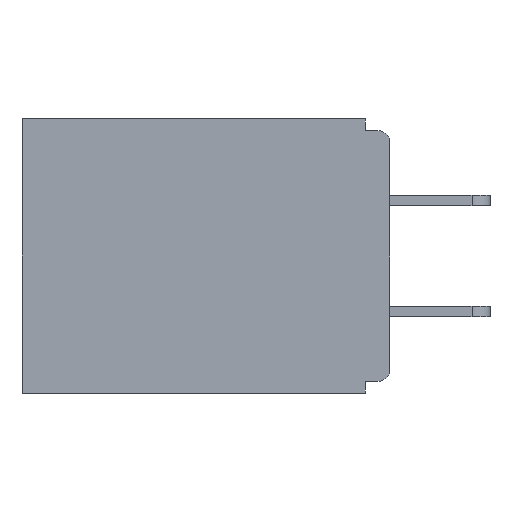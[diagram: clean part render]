
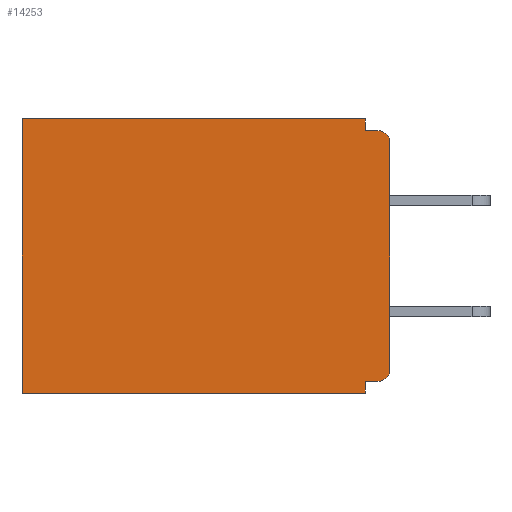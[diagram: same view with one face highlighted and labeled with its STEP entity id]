
A CAD part, left-side view. The second image highlights one B-rep face of the part: STEP entity #14253.
In plain terms, the highlighted planar face has unit normal (-1, 0, 0).
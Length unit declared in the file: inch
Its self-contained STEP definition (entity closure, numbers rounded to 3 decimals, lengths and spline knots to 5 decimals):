
#71 = VECTOR ( 'NONE', #6098, 39.37008 ) ;
#136 = LINE ( 'NONE', #7848, #893 ) ;
#165 = VECTOR ( 'NONE', #1914, 39.37008 ) ;
#212 = CARTESIAN_POINT ( 'NONE',  ( 0.298, 0.015, -0.313 ) ) ;
#882 = ORIENTED_EDGE ( 'NONE', *, *, #3048, .T. ) ;
#893 = VECTOR ( 'NONE', #1879, 39.37008 ) ;
#939 = EDGE_CURVE ( 'NONE', #12986, #13128, #13913, .T. ) ;
#944 = VERTEX_POINT ( 'NONE', #994 ) ;
#994 = CARTESIAN_POINT ( 'NONE',  ( 0.298, 0.031, 0. ) ) ;
#1046 = EDGE_CURVE ( 'NONE', #944, #14890, #9510, .T. ) ;
#1520 = CARTESIAN_POINT ( 'NONE',  ( 0.298, 0.46, 0. ) ) ;
#1879 = DIRECTION ( 'NONE',  ( 0., 0., -1. ) ) ;
#1914 = DIRECTION ( 'NONE',  ( 0., 1., 0. ) ) ;
#2322 = VERTEX_POINT ( 'NONE', #11423 ) ;
#2573 = CARTESIAN_POINT ( 'NONE',  ( 0.298, 0.015, -0.328 ) ) ;
#2696 = DIRECTION ( 'NONE',  ( 1., 0., 0. ) ) ;
#2762 = VERTEX_POINT ( 'NONE', #11444 ) ;
#2806 = PLANE ( 'NONE',  #10597 ) ;
#2978 = DIRECTION ( 'NONE',  ( 0., 0., -1. ) ) ;
#3048 = EDGE_CURVE ( 'NONE', #14890, #8709, #12552, .T. ) ;
#3119 = CARTESIAN_POINT ( 'NONE',  ( 0.298, 0.031, -0.015 ) ) ;
#3135 = VECTOR ( 'NONE', #13973, 39.37008 ) ;
#3329 = ORIENTED_EDGE ( 'NONE', *, *, #3625, .F. ) ;
#3625 = EDGE_CURVE ( 'NONE', #5323, #8709, #9414, .T. ) ;
#3799 = AXIS2_PLACEMENT_3D ( 'NONE', #212, #12065, #4925 ) ;
#3844 = ORIENTED_EDGE ( 'NONE', *, *, #5430, .F. ) ;
#3948 = VERTEX_POINT ( 'NONE', #3119 ) ;
#3999 = DIRECTION ( 'NONE',  ( 0., 0., -1. ) ) ;
#4664 = CARTESIAN_POINT ( 'NONE',  ( 0.298, 0., -0.328 ) ) ;
#4867 = EDGE_LOOP ( 'NONE', ( #12071, #6610, #3844, #10008, #882, #3329, #11223, #5649, #13208, #8005 ) ) ;
#4925 = DIRECTION ( 'NONE',  ( 0., 0., -1. ) ) ;
#4975 = VECTOR ( 'NONE', #2978, 39.37008 ) ;
#5263 = DIRECTION ( 'NONE',  ( 0., 0., -1. ) ) ;
#5323 = VERTEX_POINT ( 'NONE', #8236 ) ;
#5430 = EDGE_CURVE ( 'NONE', #944, #3948, #6997, .T. ) ;
#5561 = FACE_OUTER_BOUND ( 'NONE', #4867, .T. ) ;
#5637 = EDGE_CURVE ( 'NONE', #12986, #2322, #136, .T. ) ;
#5649 = ORIENTED_EDGE ( 'NONE', *, *, #6223, .F. ) ;
#5997 = CARTESIAN_POINT ( 'NONE',  ( 0.298, 0., 0. ) ) ;
#6098 = DIRECTION ( 'NONE',  ( 0., 1., 0. ) ) ;
#6223 = EDGE_CURVE ( 'NONE', #11171, #2762, #10090, .T. ) ;
#6610 = ORIENTED_EDGE ( 'NONE', *, *, #9377, .F. ) ;
#6997 = LINE ( 'NONE', #7966, #4975 ) ;
#7439 = AXIS2_PLACEMENT_3D ( 'NONE', #11352, #12903, #15234 ) ;
#7456 = LINE ( 'NONE', #14657, #8204 ) ;
#7722 = VECTOR ( 'NONE', #12890, 39.37008 ) ;
#7829 = CARTESIAN_POINT ( 'NONE',  ( 0.298, 0., -0.343 ) ) ;
#7848 = CARTESIAN_POINT ( 'NONE',  ( 0.298, 0., 0. ) ) ;
#7871 = CIRCLE ( 'NONE', #3799, 0.015 ) ;
#7966 = CARTESIAN_POINT ( 'NONE',  ( 0.298, 0.031, -0.343 ) ) ;
#8005 = ORIENTED_EDGE ( 'NONE', *, *, #5637, .F. ) ;
#8204 = VECTOR ( 'NONE', #12473, 39.37008 ) ;
#8236 = CARTESIAN_POINT ( 'NONE',  ( 0.298, 0.031, -0.343 ) ) ;
#8709 = VERTEX_POINT ( 'NONE', #14580 ) ;
#8730 = CARTESIAN_POINT ( 'NONE',  ( 0.298, 0.031, -0.343 ) ) ;
#8783 = LINE ( 'NONE', #8730, #9869 ) ;
#8897 = EDGE_CURVE ( 'NONE', #2762, #5323, #8783, .T. ) ;
#9377 = EDGE_CURVE ( 'NONE', #3948, #13128, #7456, .T. ) ;
#9414 = LINE ( 'NONE', #7829, #165 ) ;
#9471 = CARTESIAN_POINT ( 'NONE',  ( 0.298, 0.015, -0.015 ) ) ;
#9510 = LINE ( 'NONE', #5997, #71 ) ;
#9869 = VECTOR ( 'NONE', #5263, 39.37008 ) ;
#10008 = ORIENTED_EDGE ( 'NONE', *, *, #1046, .T. ) ;
#10090 = LINE ( 'NONE', #4664, #7722 ) ;
#10533 = CARTESIAN_POINT ( 'NONE',  ( 0.298, 0.46, 0. ) ) ;
#10597 = AXIS2_PLACEMENT_3D ( 'NONE', #13275, #2696, #3999 ) ;
#11050 = EDGE_CURVE ( 'NONE', #11171, #2322, #7871, .T. ) ;
#11171 = VERTEX_POINT ( 'NONE', #2573 ) ;
#11223 = ORIENTED_EDGE ( 'NONE', *, *, #8897, .F. ) ;
#11352 = CARTESIAN_POINT ( 'NONE',  ( 0.298, 0.015, -0.03 ) ) ;
#11423 = CARTESIAN_POINT ( 'NONE',  ( 0.298, 0., -0.313 ) ) ;
#11444 = CARTESIAN_POINT ( 'NONE',  ( 0.298, 0.031, -0.328 ) ) ;
#11832 = CARTESIAN_POINT ( 'NONE',  ( 0.298, 0., -0.03 ) ) ;
#12065 = DIRECTION ( 'NONE',  ( -1., 0., 0. ) ) ;
#12071 = ORIENTED_EDGE ( 'NONE', *, *, #939, .T. ) ;
#12473 = DIRECTION ( 'NONE',  ( 0., -1., 0. ) ) ;
#12552 = LINE ( 'NONE', #10533, #3135 ) ;
#12890 = DIRECTION ( 'NONE',  ( 0., 1., 0. ) ) ;
#12903 = DIRECTION ( 'NONE',  ( -1., 0., 0. ) ) ;
#12986 = VERTEX_POINT ( 'NONE', #11832 ) ;
#13128 = VERTEX_POINT ( 'NONE', #9471 ) ;
#13208 = ORIENTED_EDGE ( 'NONE', *, *, #11050, .T. ) ;
#13275 = CARTESIAN_POINT ( 'NONE',  ( 0.298, 0., 0. ) ) ;
#13913 = CIRCLE ( 'NONE', #7439, 0.015 ) ;
#13973 = DIRECTION ( 'NONE',  ( 0., 0., -1. ) ) ;
#14253 = ADVANCED_FACE ( 'NONE', ( #5561 ), #2806, .F. ) ;
#14580 = CARTESIAN_POINT ( 'NONE',  ( 0.298, 0.46, -0.343 ) ) ;
#14657 = CARTESIAN_POINT ( 'NONE',  ( 0.298, 0., -0.015 ) ) ;
#14890 = VERTEX_POINT ( 'NONE', #1520 ) ;
#15234 = DIRECTION ( 'NONE',  ( 0., 0., -1. ) ) ;
